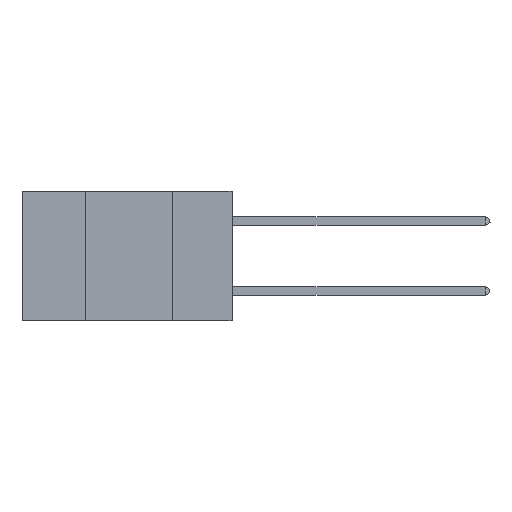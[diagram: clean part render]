
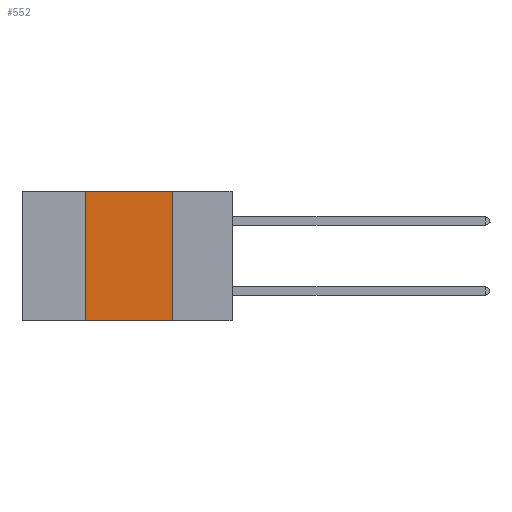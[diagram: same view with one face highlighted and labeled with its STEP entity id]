
A CAD part, left-side view. The second image highlights one B-rep face of the part: STEP entity #552.
In plain terms, the highlighted planar face has unit normal (-1, 0, 0).
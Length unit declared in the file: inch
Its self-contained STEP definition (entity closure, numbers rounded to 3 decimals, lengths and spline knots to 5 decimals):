
#301 = PLANE ( 'NONE',  #18044 ) ;
#552 = ADVANCED_FACE ( 'NONE', ( #16101 ), #301, .F. ) ;
#944 = LINE ( 'NONE', #4449, #7962 ) ;
#1018 = LINE ( 'NONE', #10965, #11762 ) ;
#1404 = DIRECTION ( 'NONE',  ( 1., 0., 0. ) ) ;
#1604 = EDGE_CURVE ( 'NONE', #17794, #13240, #13880, .T. ) ;
#2504 = DIRECTION ( 'NONE',  ( 0., 0., -1. ) ) ;
#4139 = CARTESIAN_POINT ( 'NONE',  ( 0., 0.42, -0.37 ) ) ;
#4449 = CARTESIAN_POINT ( 'NONE',  ( 0., 0.6, -0.37 ) ) ;
#4671 = VECTOR ( 'NONE', #15044, 39.37008 ) ;
#5388 = CARTESIAN_POINT ( 'NONE',  ( 0., 0.42, 0. ) ) ;
#6008 = EDGE_CURVE ( 'NONE', #13240, #11902, #15146, .T. ) ;
#6319 = EDGE_LOOP ( 'NONE', ( #8966, #20393, #10365, #6622 ) ) ;
#6622 = ORIENTED_EDGE ( 'NONE', *, *, #14730, .T. ) ;
#6741 = VECTOR ( 'NONE', #13654, 39.37008 ) ;
#7921 = DIRECTION ( 'NONE',  ( 0., 0., -1. ) ) ;
#7962 = VECTOR ( 'NONE', #18841, 39.37008 ) ;
#8563 = VERTEX_POINT ( 'NONE', #13171 ) ;
#8966 = ORIENTED_EDGE ( 'NONE', *, *, #18354, .F. ) ;
#9150 = CARTESIAN_POINT ( 'NONE',  ( 0., 0.17, 0. ) ) ;
#10365 = ORIENTED_EDGE ( 'NONE', *, *, #1604, .F. ) ;
#10965 = CARTESIAN_POINT ( 'NONE',  ( 0., 0.17, 0. ) ) ;
#11762 = VECTOR ( 'NONE', #2504, 39.37008 ) ;
#11902 = VERTEX_POINT ( 'NONE', #9150 ) ;
#13171 = CARTESIAN_POINT ( 'NONE',  ( 0., 0.17, -0.37 ) ) ;
#13240 = VERTEX_POINT ( 'NONE', #18912 ) ;
#13654 = DIRECTION ( 'NONE',  ( 0., 0., 1. ) ) ;
#13880 = LINE ( 'NONE', #5388, #6741 ) ;
#14730 = EDGE_CURVE ( 'NONE', #17794, #8563, #944, .T. ) ;
#15044 = DIRECTION ( 'NONE',  ( 0., -1., 0. ) ) ;
#15146 = LINE ( 'NONE', #16542, #4671 ) ;
#16010 = CARTESIAN_POINT ( 'NONE',  ( 0., 0.6, 0. ) ) ;
#16101 = FACE_OUTER_BOUND ( 'NONE', #6319, .T. ) ;
#16542 = CARTESIAN_POINT ( 'NONE',  ( 0., 0.6, 0. ) ) ;
#17794 = VERTEX_POINT ( 'NONE', #4139 ) ;
#18044 = AXIS2_PLACEMENT_3D ( 'NONE', #16010, #1404, #7921 ) ;
#18354 = EDGE_CURVE ( 'NONE', #11902, #8563, #1018, .T. ) ;
#18841 = DIRECTION ( 'NONE',  ( 0., -1., 0. ) ) ;
#18912 = CARTESIAN_POINT ( 'NONE',  ( 0., 0.42, 0. ) ) ;
#20393 = ORIENTED_EDGE ( 'NONE', *, *, #6008, .F. ) ;
